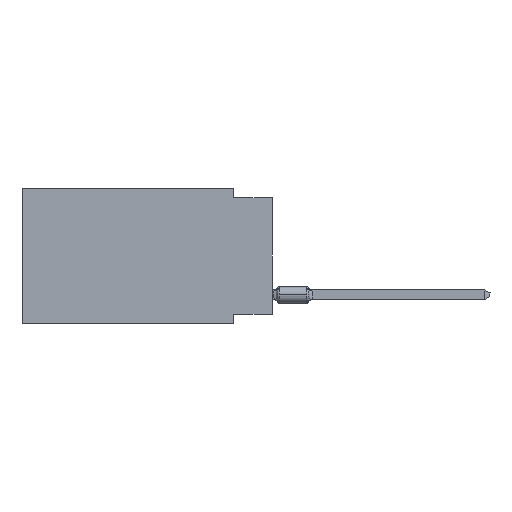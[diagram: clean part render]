
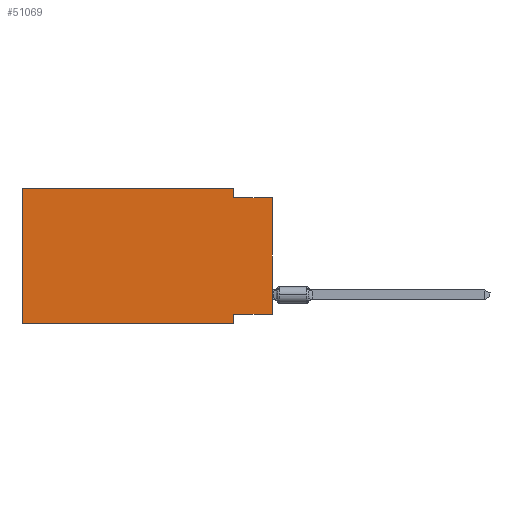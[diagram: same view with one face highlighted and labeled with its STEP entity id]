
A CAD part, left-side view. The second image highlights one B-rep face of the part: STEP entity #51069.
In plain terms, the highlighted planar face has unit normal (-1, 0, 0).
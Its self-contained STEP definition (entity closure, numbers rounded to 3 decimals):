
#2073 = VERTEX_POINT ( 'NONE', #42567 ) ;
#3340 = EDGE_CURVE ( 'NONE', #7835, #72233, #61207, .T. ) ;
#3436 = CARTESIAN_POINT ( 'NONE',  ( 0., 16.383, -8.89 ) ) ;
#7835 = VERTEX_POINT ( 'NONE', #26600 ) ;
#9326 = CARTESIAN_POINT ( 'NONE',  ( 0., 2.54, -0.635 ) ) ;
#10141 = DIRECTION ( 'NONE',  ( 0., 0., -1. ) ) ;
#11794 = CARTESIAN_POINT ( 'NONE',  ( 0., 2.54, -8.89 ) ) ;
#12206 = VERTEX_POINT ( 'NONE', #49300 ) ;
#12664 = LINE ( 'NONE', #37819, #47263 ) ;
#13810 = CARTESIAN_POINT ( 'NONE',  ( 0., 2.54, -8.89 ) ) ;
#13928 = DIRECTION ( 'NONE',  ( 0., -1., 0. ) ) ;
#14806 = CARTESIAN_POINT ( 'NONE',  ( 0., 16.383, -8.89 ) ) ;
#15314 = PLANE ( 'NONE',  #54967 ) ;
#19120 = CARTESIAN_POINT ( 'NONE',  ( 0., 16.383, 0. ) ) ;
#20425 = VECTOR ( 'NONE', #79226, 1000. ) ;
#21125 = FACE_OUTER_BOUND ( 'NONE', #80544, .T. ) ;
#22051 = EDGE_CURVE ( 'NONE', #74827, #2073, #75554, .T. ) ;
#23259 = VECTOR ( 'NONE', #10141, 1000. ) ;
#24860 = DIRECTION ( 'NONE',  ( 0., 0., 1. ) ) ;
#26237 = ORIENTED_EDGE ( 'NONE', *, *, #64361, .F. ) ;
#26254 = VECTOR ( 'NONE', #45909, 1000. ) ;
#26600 = CARTESIAN_POINT ( 'NONE',  ( 0., 2.54, 0. ) ) ;
#29441 = CARTESIAN_POINT ( 'NONE',  ( 0., 16.383, 0. ) ) ;
#31545 = VERTEX_POINT ( 'NONE', #13810 ) ;
#32491 = CARTESIAN_POINT ( 'NONE',  ( 0., 0., -0.635 ) ) ;
#33920 = VERTEX_POINT ( 'NONE', #60950 ) ;
#34196 = EDGE_CURVE ( 'NONE', #2073, #7835, #54959, .T. ) ;
#37819 = CARTESIAN_POINT ( 'NONE',  ( 0., 0., -8.255 ) ) ;
#40078 = VECTOR ( 'NONE', #53373, 1000. ) ;
#41582 = VECTOR ( 'NONE', #49701, 1000. ) ;
#41659 = ORIENTED_EDGE ( 'NONE', *, *, #34196, .F. ) ;
#42157 = LINE ( 'NONE', #3436, #20425 ) ;
#42324 = LINE ( 'NONE', #11794, #41582 ) ;
#42567 = CARTESIAN_POINT ( 'NONE',  ( 0., 16.383, 0. ) ) ;
#45909 = DIRECTION ( 'NONE',  ( 0., 0., 1. ) ) ;
#46270 = CARTESIAN_POINT ( 'NONE',  ( 0., 16.383, 0. ) ) ;
#47263 = VECTOR ( 'NONE', #48552, 1000. ) ;
#47467 = DIRECTION ( 'NONE',  ( 0., 0., -1. ) ) ;
#48103 = EDGE_CURVE ( 'NONE', #33920, #57744, #56580, .T. ) ;
#48552 = DIRECTION ( 'NONE',  ( 0., 1., 0. ) ) ;
#49300 = CARTESIAN_POINT ( 'NONE',  ( 0., 2.54, -8.255 ) ) ;
#49701 = DIRECTION ( 'NONE',  ( 0., 0., -1. ) ) ;
#50182 = ORIENTED_EDGE ( 'NONE', *, *, #3340, .F. ) ;
#50487 = EDGE_CURVE ( 'NONE', #72233, #57744, #63776, .T. ) ;
#51069 = ADVANCED_FACE ( 'NONE', ( #21125 ), #15314, .F. ) ;
#51213 = CARTESIAN_POINT ( 'NONE',  ( 0., 0., 0. ) ) ;
#53373 = DIRECTION ( 'NONE',  ( 0., -1., 0. ) ) ;
#54959 = LINE ( 'NONE', #29441, #40078 ) ;
#54967 = AXIS2_PLACEMENT_3D ( 'NONE', #46270, #79159, #47467 ) ;
#56307 = ORIENTED_EDGE ( 'NONE', *, *, #48103, .T. ) ;
#56580 = LINE ( 'NONE', #51213, #68376 ) ;
#57744 = VERTEX_POINT ( 'NONE', #63274 ) ;
#60950 = CARTESIAN_POINT ( 'NONE',  ( 0., 0., -8.255 ) ) ;
#61207 = LINE ( 'NONE', #66585, #23259 ) ;
#61504 = VECTOR ( 'NONE', #13928, 1000. ) ;
#62068 = EDGE_CURVE ( 'NONE', #12206, #31545, #42324, .T. ) ;
#63274 = CARTESIAN_POINT ( 'NONE',  ( 0., 0., -0.635 ) ) ;
#63776 = LINE ( 'NONE', #32491, #61504 ) ;
#64361 = EDGE_CURVE ( 'NONE', #33920, #12206, #12664, .T. ) ;
#65786 = ORIENTED_EDGE ( 'NONE', *, *, #62068, .F. ) ;
#66585 = CARTESIAN_POINT ( 'NONE',  ( 0., 2.54, 0. ) ) ;
#67673 = EDGE_CURVE ( 'NONE', #74827, #31545, #42157, .T. ) ;
#68376 = VECTOR ( 'NONE', #24860, 1000. ) ;
#68937 = ORIENTED_EDGE ( 'NONE', *, *, #67673, .T. ) ;
#72233 = VERTEX_POINT ( 'NONE', #9326 ) ;
#72617 = ORIENTED_EDGE ( 'NONE', *, *, #22051, .F. ) ;
#74827 = VERTEX_POINT ( 'NONE', #14806 ) ;
#75554 = LINE ( 'NONE', #19120, #26254 ) ;
#79159 = DIRECTION ( 'NONE',  ( 1., 0., 0. ) ) ;
#79226 = DIRECTION ( 'NONE',  ( 0., -1., 0. ) ) ;
#80016 = ORIENTED_EDGE ( 'NONE', *, *, #50487, .F. ) ;
#80544 = EDGE_LOOP ( 'NONE', ( #56307, #80016, #50182, #41659, #72617, #68937, #65786, #26237 ) ) ;
